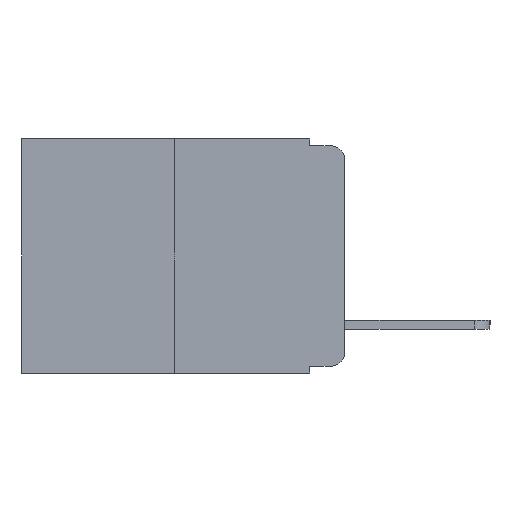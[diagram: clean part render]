
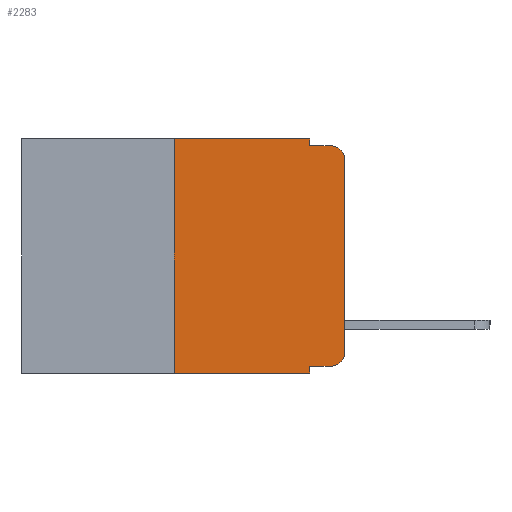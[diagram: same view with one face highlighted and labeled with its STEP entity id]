
A CAD part, left-side view. The second image highlights one B-rep face of the part: STEP entity #2283.
In plain terms, the highlighted planar face has unit normal (-1, 0, 0).
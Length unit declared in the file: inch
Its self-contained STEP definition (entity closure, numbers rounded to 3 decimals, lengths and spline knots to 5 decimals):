
#63 = CARTESIAN_POINT ( 'NONE',  ( 0., 0., -0.313 ) ) ;
#141 = LINE ( 'NONE', #3312, #12473 ) ;
#216 = VERTEX_POINT ( 'NONE', #15265 ) ;
#416 = DIRECTION ( 'NONE',  ( 0., 0., -1. ) ) ;
#529 = ORIENTED_EDGE ( 'NONE', *, *, #18376, .T. ) ;
#655 = CARTESIAN_POINT ( 'NONE',  ( 0., 0.25, 0. ) ) ;
#842 = CIRCLE ( 'NONE', #5694, 0.02 ) ;
#846 = EDGE_CURVE ( 'NONE', #6611, #14369, #4134, .T. ) ;
#1296 = VERTEX_POINT ( 'NONE', #10161 ) ;
#1297 = VERTEX_POINT ( 'NONE', #63 ) ;
#1634 = CARTESIAN_POINT ( 'NONE',  ( 0., 0.25, -0.343 ) ) ;
#1936 = CARTESIAN_POINT ( 'NONE',  ( 0., 0.051, -0.343 ) ) ;
#2283 = ADVANCED_FACE ( 'NONE', ( #3299 ), #7557, .F. ) ;
#2731 = VERTEX_POINT ( 'NONE', #1936 ) ;
#2853 = LINE ( 'NONE', #4189, #12609 ) ;
#3084 = CARTESIAN_POINT ( 'NONE',  ( 0., 0.25, 0. ) ) ;
#3299 = FACE_OUTER_BOUND ( 'NONE', #9527, .T. ) ;
#3312 = CARTESIAN_POINT ( 'NONE',  ( 0., 0.051, -0.01 ) ) ;
#3405 = VECTOR ( 'NONE', #17227, 39.37008 ) ;
#3607 = AXIS2_PLACEMENT_3D ( 'NONE', #3656, #12273, #16825 ) ;
#3635 = CARTESIAN_POINT ( 'NONE',  ( 0., 0., -0.03 ) ) ;
#3656 = CARTESIAN_POINT ( 'NONE',  ( 0., 0.02, -0.313 ) ) ;
#4134 = LINE ( 'NONE', #14244, #3405 ) ;
#4189 = CARTESIAN_POINT ( 'NONE',  ( 0., 0.473, 0. ) ) ;
#4235 = ORIENTED_EDGE ( 'NONE', *, *, #8524, .T. ) ;
#4483 = ORIENTED_EDGE ( 'NONE', *, *, #4498, .F. ) ;
#4498 = EDGE_CURVE ( 'NONE', #14369, #216, #141, .T. ) ;
#5070 = VERTEX_POINT ( 'NONE', #6305 ) ;
#5571 = VECTOR ( 'NONE', #11190, 39.37008 ) ;
#5694 = AXIS2_PLACEMENT_3D ( 'NONE', #16367, #8860, #13386 ) ;
#6120 = DIRECTION ( 'NONE',  ( 0., -1., 0. ) ) ;
#6200 = VECTOR ( 'NONE', #6120, 39.37008 ) ;
#6305 = CARTESIAN_POINT ( 'NONE',  ( 0., 0.02, -0.333 ) ) ;
#6320 = LINE ( 'NONE', #16852, #17722 ) ;
#6401 = CARTESIAN_POINT ( 'NONE',  ( 0., 0.473, 0. ) ) ;
#6611 = VERTEX_POINT ( 'NONE', #16938 ) ;
#6995 = ORIENTED_EDGE ( 'NONE', *, *, #11131, .F. ) ;
#7303 = VERTEX_POINT ( 'NONE', #655 ) ;
#7557 = PLANE ( 'NONE',  #10714 ) ;
#7731 = DIRECTION ( 'NONE',  ( 0., 0., 1. ) ) ;
#7985 = VECTOR ( 'NONE', #7731, 39.37008 ) ;
#8277 = ORIENTED_EDGE ( 'NONE', *, *, #14187, .T. ) ;
#8281 = CARTESIAN_POINT ( 'NONE',  ( 0., 0.051, -0.01 ) ) ;
#8468 = CARTESIAN_POINT ( 'NONE',  ( 0., 0.051, 0. ) ) ;
#8502 = VERTEX_POINT ( 'NONE', #3635 ) ;
#8524 = EDGE_CURVE ( 'NONE', #1296, #5070, #16981, .T. ) ;
#8860 = DIRECTION ( 'NONE',  ( -1., 0., 0. ) ) ;
#9406 = EDGE_CURVE ( 'NONE', #1297, #8502, #6320, .T. ) ;
#9513 = CARTESIAN_POINT ( 'NONE',  ( 0., 0.051, -0.333 ) ) ;
#9527 = EDGE_LOOP ( 'NONE', ( #17291, #9798, #4483, #14779, #10661, #14463, #529, #6995, #4235, #8277 ) ) ;
#9798 = ORIENTED_EDGE ( 'NONE', *, *, #14066, .T. ) ;
#10063 = LINE ( 'NONE', #8468, #14721 ) ;
#10161 = CARTESIAN_POINT ( 'NONE',  ( 0., 0.051, -0.333 ) ) ;
#10661 = ORIENTED_EDGE ( 'NONE', *, *, #11008, .F. ) ;
#10714 = AXIS2_PLACEMENT_3D ( 'NONE', #6401, #17709, #416 ) ;
#11008 = EDGE_CURVE ( 'NONE', #7303, #6611, #2853, .T. ) ;
#11131 = EDGE_CURVE ( 'NONE', #1296, #2731, #10063, .T. ) ;
#11190 = DIRECTION ( 'NONE',  ( 0., -1., 0. ) ) ;
#11549 = VERTEX_POINT ( 'NONE', #1634 ) ;
#12005 = CARTESIAN_POINT ( 'NONE',  ( 0., 0.473, -0.343 ) ) ;
#12092 = LINE ( 'NONE', #3084, #7985 ) ;
#12273 = DIRECTION ( 'NONE',  ( -1., 0., 0. ) ) ;
#12303 = DIRECTION ( 'NONE',  ( 0., 0., 1. ) ) ;
#12473 = VECTOR ( 'NONE', #16206, 39.37008 ) ;
#12609 = VECTOR ( 'NONE', #17478, 39.37008 ) ;
#12939 = CIRCLE ( 'NONE', #3607, 0.02 ) ;
#13314 = LINE ( 'NONE', #12005, #6200 ) ;
#13386 = DIRECTION ( 'NONE',  ( 0., 0., -1. ) ) ;
#14066 = EDGE_CURVE ( 'NONE', #8502, #216, #842, .T. ) ;
#14187 = EDGE_CURVE ( 'NONE', #5070, #1297, #12939, .T. ) ;
#14215 = DIRECTION ( 'NONE',  ( 0., 0., -1. ) ) ;
#14244 = CARTESIAN_POINT ( 'NONE',  ( 0., 0.051, 0. ) ) ;
#14369 = VERTEX_POINT ( 'NONE', #8281 ) ;
#14463 = ORIENTED_EDGE ( 'NONE', *, *, #15880, .F. ) ;
#14721 = VECTOR ( 'NONE', #14215, 39.37008 ) ;
#14779 = ORIENTED_EDGE ( 'NONE', *, *, #846, .F. ) ;
#15265 = CARTESIAN_POINT ( 'NONE',  ( 0., 0.02, -0.01 ) ) ;
#15880 = EDGE_CURVE ( 'NONE', #11549, #7303, #12092, .T. ) ;
#16206 = DIRECTION ( 'NONE',  ( 0., -1., 0. ) ) ;
#16367 = CARTESIAN_POINT ( 'NONE',  ( 0., 0.02, -0.03 ) ) ;
#16825 = DIRECTION ( 'NONE',  ( 0., 0., -1. ) ) ;
#16852 = CARTESIAN_POINT ( 'NONE',  ( 0., 0., 0. ) ) ;
#16938 = CARTESIAN_POINT ( 'NONE',  ( 0., 0.051, 0. ) ) ;
#16981 = LINE ( 'NONE', #9513, #5571 ) ;
#17227 = DIRECTION ( 'NONE',  ( 0., 0., -1. ) ) ;
#17291 = ORIENTED_EDGE ( 'NONE', *, *, #9406, .T. ) ;
#17478 = DIRECTION ( 'NONE',  ( 0., -1., 0. ) ) ;
#17709 = DIRECTION ( 'NONE',  ( 1., 0., 0. ) ) ;
#17722 = VECTOR ( 'NONE', #12303, 39.37008 ) ;
#18376 = EDGE_CURVE ( 'NONE', #11549, #2731, #13314, .T. ) ;
